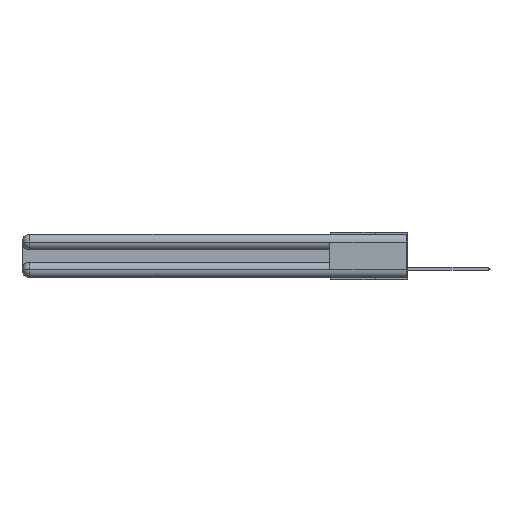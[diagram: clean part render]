
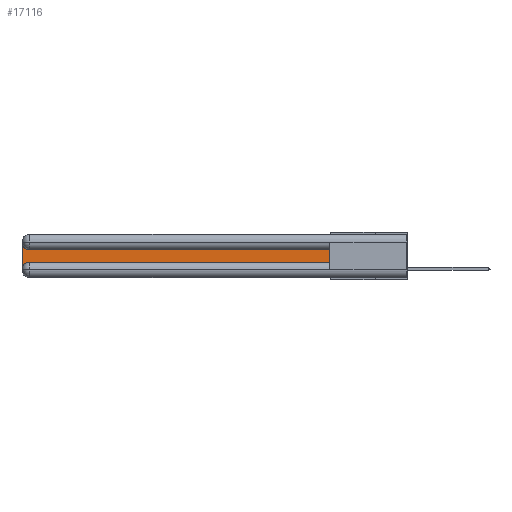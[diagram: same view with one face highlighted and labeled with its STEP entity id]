
A CAD part, left-side view. The second image highlights one B-rep face of the part: STEP entity #17116.
In plain terms, the highlighted planar face has unit normal (-1, 0, 0).
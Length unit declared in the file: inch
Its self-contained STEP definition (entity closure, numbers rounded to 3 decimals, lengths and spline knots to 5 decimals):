
#41 = EDGE_LOOP ( 'NONE', ( #3194, #6674, #25299, #1489, #8578, #13416 ) ) ;
#704 = CARTESIAN_POINT ( 'NONE',  ( 0.075, 2.94, -0.1225 ) ) ;
#1034 = CARTESIAN_POINT ( 'NONE',  ( 0.075, 0.6, -0.2175 ) ) ;
#1473 = DIRECTION ( 'NONE',  ( 1., 0., 0. ) ) ;
#1489 = ORIENTED_EDGE ( 'NONE', *, *, #10566, .T. ) ;
#1959 = PLANE ( 'NONE',  #3448 ) ;
#2868 = EDGE_CURVE ( 'NONE', #3318, #3642, #23881, .T. ) ;
#2886 = CIRCLE ( 'NONE', #17842, 0.06 ) ;
#3045 = DIRECTION ( 'NONE',  ( 0., 1., 0. ) ) ;
#3194 = ORIENTED_EDGE ( 'NONE', *, *, #21565, .T. ) ;
#3318 = VERTEX_POINT ( 'NONE', #10234 ) ;
#3448 = AXIS2_PLACEMENT_3D ( 'NONE', #28661, #10435, #26395 ) ;
#3642 = VERTEX_POINT ( 'NONE', #27532 ) ;
#5216 = DIRECTION ( 'NONE',  ( 0., 0., -1. ) ) ;
#5622 = DIRECTION ( 'NONE',  ( 1., 0., 0. ) ) ;
#6674 = ORIENTED_EDGE ( 'NONE', *, *, #7437, .T. ) ;
#6718 = CARTESIAN_POINT ( 'NONE',  ( 0.075, 2.94, -0.2175 ) ) ;
#7274 = CARTESIAN_POINT ( 'NONE',  ( 0.075, 0.6, -0.2175 ) ) ;
#7437 = EDGE_CURVE ( 'NONE', #20413, #3318, #2886, .T. ) ;
#7741 = EDGE_CURVE ( 'NONE', #20976, #10307, #27817, .T. ) ;
#8084 = FACE_OUTER_BOUND ( 'NONE', #41, .T. ) ;
#8578 = ORIENTED_EDGE ( 'NONE', *, *, #20390, .T. ) ;
#8612 = LINE ( 'NONE', #15926, #10703 ) ;
#10234 = CARTESIAN_POINT ( 'NONE',  ( 0.075, 3., -0.0625 ) ) ;
#10307 = VERTEX_POINT ( 'NONE', #23274 ) ;
#10435 = DIRECTION ( 'NONE',  ( 1., 0., 0. ) ) ;
#10566 = EDGE_CURVE ( 'NONE', #3642, #24238, #16972, .T. ) ;
#10703 = VECTOR ( 'NONE', #12084, 39.37008 ) ;
#11340 = AXIS2_PLACEMENT_3D ( 'NONE', #17260, #1473, #15267 ) ;
#12084 = DIRECTION ( 'NONE',  ( 0., -1., 0. ) ) ;
#13416 = ORIENTED_EDGE ( 'NONE', *, *, #7741, .T. ) ;
#14027 = CARTESIAN_POINT ( 'NONE',  ( 0.075, 0.6, -0.1225 ) ) ;
#15009 = VECTOR ( 'NONE', #23248, 39.37008 ) ;
#15267 = DIRECTION ( 'NONE',  ( 0., 0., -1. ) ) ;
#15926 = CARTESIAN_POINT ( 'NONE',  ( 0.075, 0.6, -0.2175 ) ) ;
#16684 = DIRECTION ( 'NONE',  ( 0., 0., -1. ) ) ;
#16972 = CIRCLE ( 'NONE', #11340, 0.06 ) ;
#17116 = ADVANCED_FACE ( 'NONE', ( #8084 ), #1959, .F. ) ;
#17260 = CARTESIAN_POINT ( 'NONE',  ( 0.075, 2.94, -0.2775 ) ) ;
#17842 = AXIS2_PLACEMENT_3D ( 'NONE', #23578, #5622, #5216 ) ;
#20390 = EDGE_CURVE ( 'NONE', #24238, #20976, #8612, .T. ) ;
#20413 = VERTEX_POINT ( 'NONE', #704 ) ;
#20976 = VERTEX_POINT ( 'NONE', #1034 ) ;
#21565 = EDGE_CURVE ( 'NONE', #10307, #20413, #29191, .T. ) ;
#23248 = DIRECTION ( 'NONE',  ( 0., 0., 1. ) ) ;
#23274 = CARTESIAN_POINT ( 'NONE',  ( 0.075, 0.6, -0.1225 ) ) ;
#23544 = VECTOR ( 'NONE', #16684, 39.37008 ) ;
#23578 = CARTESIAN_POINT ( 'NONE',  ( 0.075, 2.94, -0.0625 ) ) ;
#23881 = LINE ( 'NONE', #27984, #23544 ) ;
#24238 = VERTEX_POINT ( 'NONE', #6718 ) ;
#25288 = VECTOR ( 'NONE', #3045, 39.37008 ) ;
#25299 = ORIENTED_EDGE ( 'NONE', *, *, #2868, .T. ) ;
#26395 = DIRECTION ( 'NONE',  ( 0., 0., -1. ) ) ;
#27532 = CARTESIAN_POINT ( 'NONE',  ( 0.075, 3., -0.2775 ) ) ;
#27817 = LINE ( 'NONE', #7274, #15009 ) ;
#27984 = CARTESIAN_POINT ( 'NONE',  ( 0.075, 3., -0.2175 ) ) ;
#28661 = CARTESIAN_POINT ( 'NONE',  ( 0.075, 3., -0.1225 ) ) ;
#29191 = LINE ( 'NONE', #14027, #25288 ) ;
